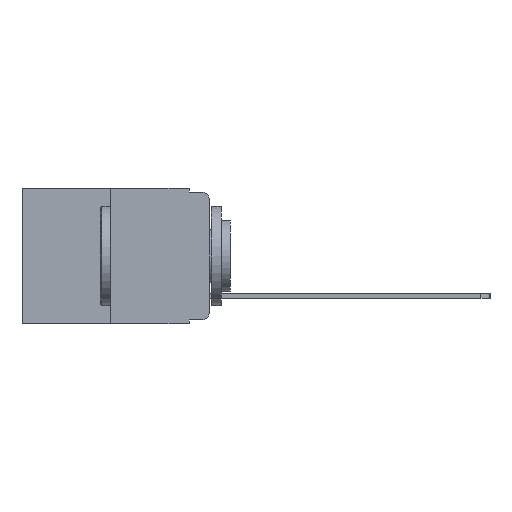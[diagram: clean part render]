
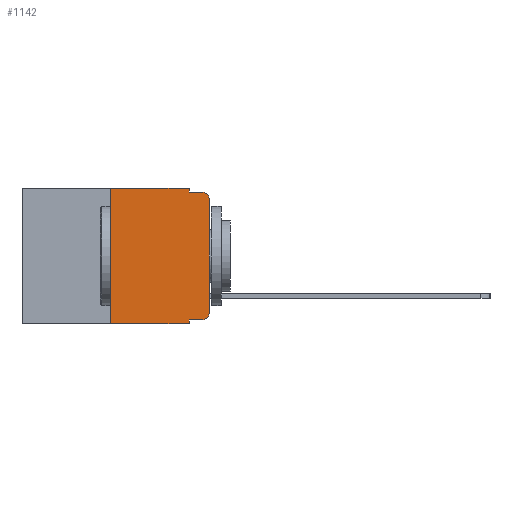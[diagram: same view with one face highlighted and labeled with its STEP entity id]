
A CAD part, left-side view. The second image highlights one B-rep face of the part: STEP entity #1142.
In plain terms, the highlighted planar face has unit normal (-1, 0, 0).
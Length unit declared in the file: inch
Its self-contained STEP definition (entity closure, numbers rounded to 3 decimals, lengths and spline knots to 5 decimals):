
#133 = VERTEX_POINT ( 'NONE', #16330 ) ;
#198 = DIRECTION ( 'NONE',  ( 1., 0., 0. ) ) ;
#328 = EDGE_CURVE ( 'NONE', #17786, #9259, #8631, .T. ) ;
#546 = ORIENTED_EDGE ( 'NONE', *, *, #1684, .F. ) ;
#595 = VERTEX_POINT ( 'NONE', #9746 ) ;
#724 = AXIS2_PLACEMENT_3D ( 'NONE', #10551, #198, #837 ) ;
#837 = DIRECTION ( 'NONE',  ( 0., 0., -1. ) ) ;
#986 = LINE ( 'NONE', #10431, #8564 ) ;
#1142 = ADVANCED_FACE ( 'NONE', ( #11821 ), #13182, .F. ) ;
#1146 = CARTESIAN_POINT ( 'NONE',  ( 0., 0.02, -0.313 ) ) ;
#1214 = CARTESIAN_POINT ( 'NONE',  ( 0., 0.02, -0.333 ) ) ;
#1320 = LINE ( 'NONE', #11720, #15613 ) ;
#1351 = LINE ( 'NONE', #13616, #4714 ) ;
#1684 = EDGE_CURVE ( 'NONE', #11284, #4924, #9380, .T. ) ;
#1836 = VERTEX_POINT ( 'NONE', #5475 ) ;
#2147 = CIRCLE ( 'NONE', #14556, 0.02 ) ;
#2367 = ORIENTED_EDGE ( 'NONE', *, *, #2988, .F. ) ;
#2499 = EDGE_CURVE ( 'NONE', #11158, #1836, #1351, .T. ) ;
#2746 = CARTESIAN_POINT ( 'NONE',  ( 0., 0.051, -0.01 ) ) ;
#2988 = EDGE_CURVE ( 'NONE', #9537, #11158, #7609, .T. ) ;
#3013 = LINE ( 'NONE', #15434, #6404 ) ;
#3193 = DIRECTION ( 'NONE',  ( -1., 0., 0. ) ) ;
#3484 = ORIENTED_EDGE ( 'NONE', *, *, #11820, .T. ) ;
#4327 = ORIENTED_EDGE ( 'NONE', *, *, #5262, .T. ) ;
#4544 = DIRECTION ( 'NONE',  ( 0., -1., 0. ) ) ;
#4714 = VECTOR ( 'NONE', #4544, 39.37008 ) ;
#4924 = VERTEX_POINT ( 'NONE', #9751 ) ;
#4973 = CARTESIAN_POINT ( 'NONE',  ( 0., 0.02, -0.03 ) ) ;
#5262 = EDGE_CURVE ( 'NONE', #7256, #17786, #986, .T. ) ;
#5294 = ORIENTED_EDGE ( 'NONE', *, *, #16181, .F. ) ;
#5330 = VECTOR ( 'NONE', #17248, 39.37008 ) ;
#5475 = CARTESIAN_POINT ( 'NONE',  ( 0., 0.051, 0. ) ) ;
#5745 = ORIENTED_EDGE ( 'NONE', *, *, #2499, .F. ) ;
#5767 = DIRECTION ( 'NONE',  ( 0., 0., 1. ) ) ;
#5897 = DIRECTION ( 'NONE',  ( 0., 0., -1. ) ) ;
#6117 = VECTOR ( 'NONE', #8603, 39.37008 ) ;
#6404 = VECTOR ( 'NONE', #5897, 39.37008 ) ;
#6441 = DIRECTION ( 'NONE',  ( 0., 0., -1. ) ) ;
#6530 = CARTESIAN_POINT ( 'NONE',  ( 0., 0.051, -0.01 ) ) ;
#6678 = ORIENTED_EDGE ( 'NONE', *, *, #17587, .T. ) ;
#7256 = VERTEX_POINT ( 'NONE', #12080 ) ;
#7609 = LINE ( 'NONE', #10936, #14402 ) ;
#8088 = CARTESIAN_POINT ( 'NONE',  ( 0., 0.25, -0.343 ) ) ;
#8418 = VECTOR ( 'NONE', #5767, 39.37008 ) ;
#8433 = DIRECTION ( 'NONE',  ( 0., 0., 1. ) ) ;
#8537 = EDGE_LOOP ( 'NONE', ( #16715, #3484, #546, #5294, #5745, #2367, #6678, #14330, #4327, #16464 ) ) ;
#8564 = VECTOR ( 'NONE', #11024, 39.37008 ) ;
#8603 = DIRECTION ( 'NONE',  ( 0., -1., 0. ) ) ;
#8631 = CIRCLE ( 'NONE', #9174, 0.02 ) ;
#9174 = AXIS2_PLACEMENT_3D ( 'NONE', #1146, #3193, #15740 ) ;
#9259 = VERTEX_POINT ( 'NONE', #11756 ) ;
#9302 = LINE ( 'NONE', #15257, #8418 ) ;
#9380 = LINE ( 'NONE', #2746, #6117 ) ;
#9537 = VERTEX_POINT ( 'NONE', #8088 ) ;
#9746 = CARTESIAN_POINT ( 'NONE',  ( 0., 0., -0.03 ) ) ;
#9751 = CARTESIAN_POINT ( 'NONE',  ( 0., 0.02, -0.01 ) ) ;
#10431 = CARTESIAN_POINT ( 'NONE',  ( 0., 0.051, -0.333 ) ) ;
#10551 = CARTESIAN_POINT ( 'NONE',  ( 0., 0.473, 0. ) ) ;
#10936 = CARTESIAN_POINT ( 'NONE',  ( 0., 0.25, 0. ) ) ;
#11024 = DIRECTION ( 'NONE',  ( 0., -1., 0. ) ) ;
#11158 = VERTEX_POINT ( 'NONE', #15794 ) ;
#11284 = VERTEX_POINT ( 'NONE', #6530 ) ;
#11720 = CARTESIAN_POINT ( 'NONE',  ( 0., 0.051, 0. ) ) ;
#11756 = CARTESIAN_POINT ( 'NONE',  ( 0., 0., -0.313 ) ) ;
#11820 = EDGE_CURVE ( 'NONE', #595, #4924, #2147, .T. ) ;
#11821 = FACE_OUTER_BOUND ( 'NONE', #8537, .T. ) ;
#12080 = CARTESIAN_POINT ( 'NONE',  ( 0., 0.051, -0.333 ) ) ;
#12715 = EDGE_CURVE ( 'NONE', #7256, #133, #3013, .T. ) ;
#13182 = PLANE ( 'NONE',  #724 ) ;
#13616 = CARTESIAN_POINT ( 'NONE',  ( 0., 0.473, 0. ) ) ;
#14330 = ORIENTED_EDGE ( 'NONE', *, *, #12715, .F. ) ;
#14402 = VECTOR ( 'NONE', #8433, 39.37008 ) ;
#14556 = AXIS2_PLACEMENT_3D ( 'NONE', #4973, #14601, #6441 ) ;
#14601 = DIRECTION ( 'NONE',  ( -1., 0., 0. ) ) ;
#15257 = CARTESIAN_POINT ( 'NONE',  ( 0., 0., 0. ) ) ;
#15434 = CARTESIAN_POINT ( 'NONE',  ( 0., 0.051, 0. ) ) ;
#15613 = VECTOR ( 'NONE', #15709, 39.37008 ) ;
#15709 = DIRECTION ( 'NONE',  ( 0., 0., -1. ) ) ;
#15740 = DIRECTION ( 'NONE',  ( 0., 0., -1. ) ) ;
#15777 = LINE ( 'NONE', #16005, #5330 ) ;
#15794 = CARTESIAN_POINT ( 'NONE',  ( 0., 0.25, 0. ) ) ;
#16005 = CARTESIAN_POINT ( 'NONE',  ( 0., 0.473, -0.343 ) ) ;
#16181 = EDGE_CURVE ( 'NONE', #1836, #11284, #1320, .T. ) ;
#16330 = CARTESIAN_POINT ( 'NONE',  ( 0., 0.051, -0.343 ) ) ;
#16464 = ORIENTED_EDGE ( 'NONE', *, *, #328, .T. ) ;
#16675 = EDGE_CURVE ( 'NONE', #9259, #595, #9302, .T. ) ;
#16715 = ORIENTED_EDGE ( 'NONE', *, *, #16675, .T. ) ;
#17248 = DIRECTION ( 'NONE',  ( 0., -1., 0. ) ) ;
#17587 = EDGE_CURVE ( 'NONE', #9537, #133, #15777, .T. ) ;
#17786 = VERTEX_POINT ( 'NONE', #1214 ) ;
